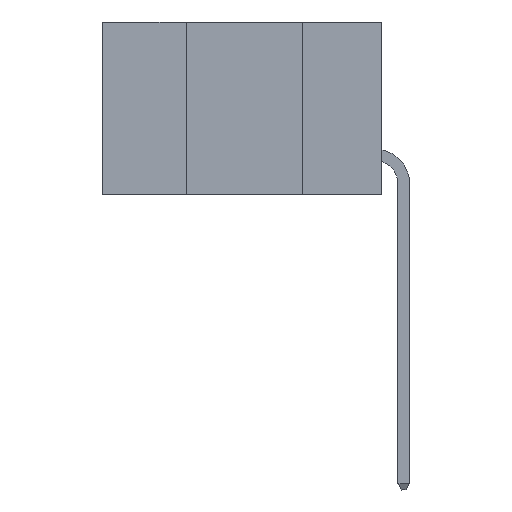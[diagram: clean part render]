
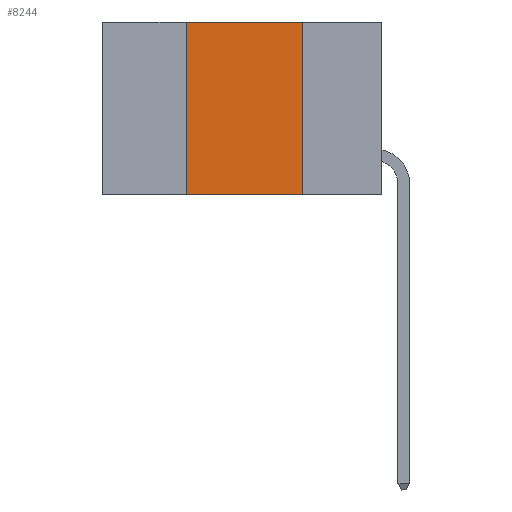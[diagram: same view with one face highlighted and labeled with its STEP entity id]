
A CAD part, left-side view. The second image highlights one B-rep face of the part: STEP entity #8244.
In plain terms, the highlighted planar face has unit normal (-1, 0, 0).
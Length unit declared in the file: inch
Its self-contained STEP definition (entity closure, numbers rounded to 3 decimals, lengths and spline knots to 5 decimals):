
#168 = ORIENTED_EDGE ( 'NONE', *, *, #22171, .F. ) ;
#1062 = DIRECTION ( 'NONE',  ( 0., -1., 0. ) ) ;
#3006 = VECTOR ( 'NONE', #1062, 39.37008 ) ;
#4352 = VERTEX_POINT ( 'NONE', #14052 ) ;
#5371 = VECTOR ( 'NONE', #13916, 39.37008 ) ;
#5760 = EDGE_CURVE ( 'NONE', #14808, #4352, #13260, .T. ) ;
#6588 = LINE ( 'NONE', #12065, #5371 ) ;
#6614 = VERTEX_POINT ( 'NONE', #17400 ) ;
#7673 = DIRECTION ( 'NONE',  ( 0., 0., 1. ) ) ;
#8244 = ADVANCED_FACE ( 'NONE', ( #12263 ), #22808, .F. ) ;
#9949 = LINE ( 'NONE', #17153, #19438 ) ;
#11477 = CARTESIAN_POINT ( 'NONE',  ( 0., 0.6, 0. ) ) ;
#11603 = EDGE_LOOP ( 'NONE', ( #15998, #24037, #168, #11914 ) ) ;
#11914 = ORIENTED_EDGE ( 'NONE', *, *, #22990, .T. ) ;
#12065 = CARTESIAN_POINT ( 'NONE',  ( 0., 0.6, -0.37 ) ) ;
#12188 = AXIS2_PLACEMENT_3D ( 'NONE', #11477, #24687, #13322 ) ;
#12263 = FACE_OUTER_BOUND ( 'NONE', #11603, .T. ) ;
#13260 = LINE ( 'NONE', #18367, #3006 ) ;
#13322 = DIRECTION ( 'NONE',  ( 0., 0., -1. ) ) ;
#13916 = DIRECTION ( 'NONE',  ( 0., -1., 0. ) ) ;
#14038 = CARTESIAN_POINT ( 'NONE',  ( 0., 0.42, -0.37 ) ) ;
#14052 = CARTESIAN_POINT ( 'NONE',  ( 0., 0.17, 0. ) ) ;
#14320 = CARTESIAN_POINT ( 'NONE',  ( 0., 0.17, 0. ) ) ;
#14808 = VERTEX_POINT ( 'NONE', #23575 ) ;
#15998 = ORIENTED_EDGE ( 'NONE', *, *, #17955, .F. ) ;
#17153 = CARTESIAN_POINT ( 'NONE',  ( 0., 0.42, 0. ) ) ;
#17400 = CARTESIAN_POINT ( 'NONE',  ( 0., 0.17, -0.37 ) ) ;
#17955 = EDGE_CURVE ( 'NONE', #4352, #6614, #19680, .T. ) ;
#18367 = CARTESIAN_POINT ( 'NONE',  ( 0., 0.6, 0. ) ) ;
#19095 = VECTOR ( 'NONE', #20002, 39.37008 ) ;
#19438 = VECTOR ( 'NONE', #7673, 39.37008 ) ;
#19680 = LINE ( 'NONE', #14320, #19095 ) ;
#20002 = DIRECTION ( 'NONE',  ( 0., 0., -1. ) ) ;
#22171 = EDGE_CURVE ( 'NONE', #24210, #14808, #9949, .T. ) ;
#22808 = PLANE ( 'NONE',  #12188 ) ;
#22990 = EDGE_CURVE ( 'NONE', #24210, #6614, #6588, .T. ) ;
#23575 = CARTESIAN_POINT ( 'NONE',  ( 0., 0.42, 0. ) ) ;
#24037 = ORIENTED_EDGE ( 'NONE', *, *, #5760, .F. ) ;
#24210 = VERTEX_POINT ( 'NONE', #14038 ) ;
#24687 = DIRECTION ( 'NONE',  ( 1., 0., 0. ) ) ;
